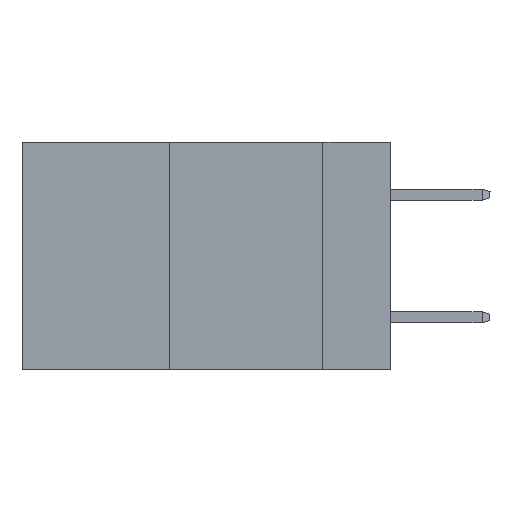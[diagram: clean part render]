
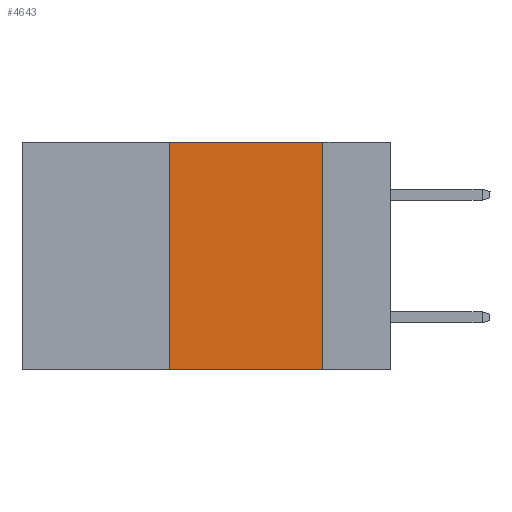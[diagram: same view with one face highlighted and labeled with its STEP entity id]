
A CAD part, left-side view. The second image highlights one B-rep face of the part: STEP entity #4643.
In plain terms, the highlighted planar face has unit normal (-1, 0, 0).
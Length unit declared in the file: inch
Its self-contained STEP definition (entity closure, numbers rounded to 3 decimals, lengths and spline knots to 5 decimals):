
#72 = DIRECTION ( 'NONE',  ( 0., -1., 0. ) ) ;
#659 = AXIS2_PLACEMENT_3D ( 'NONE', #6843, #3608, #16468 ) ;
#999 = CARTESIAN_POINT ( 'NONE',  ( 0., 0.36, -0.37 ) ) ;
#1176 = ORIENTED_EDGE ( 'NONE', *, *, #4001, .F. ) ;
#1846 = LINE ( 'NONE', #8462, #10432 ) ;
#2136 = VERTEX_POINT ( 'NONE', #12767 ) ;
#3608 = DIRECTION ( 'NONE',  ( 1., 0., 0. ) ) ;
#4001 = EDGE_CURVE ( 'NONE', #11012, #2136, #8260, .T. ) ;
#4234 = CARTESIAN_POINT ( 'NONE',  ( 0., 0.6, 0. ) ) ;
#4245 = EDGE_LOOP ( 'NONE', ( #16945, #1176, #9133, #13870 ) ) ;
#4643 = ADVANCED_FACE ( 'NONE', ( #8022 ), #15692, .F. ) ;
#5056 = VERTEX_POINT ( 'NONE', #999 ) ;
#5457 = VECTOR ( 'NONE', #6007, 39.37008 ) ;
#6007 = DIRECTION ( 'NONE',  ( 0., 0., -1. ) ) ;
#6843 = CARTESIAN_POINT ( 'NONE',  ( 0., 0.6, 0. ) ) ;
#6855 = DIRECTION ( 'NONE',  ( 0., 0., 1. ) ) ;
#7460 = DIRECTION ( 'NONE',  ( 0., -1., 0. ) ) ;
#8022 = FACE_OUTER_BOUND ( 'NONE', #4245, .T. ) ;
#8229 = EDGE_CURVE ( 'NONE', #2136, #10052, #17138, .T. ) ;
#8260 = LINE ( 'NONE', #4234, #12450 ) ;
#8462 = CARTESIAN_POINT ( 'NONE',  ( 0., 0.36, 0. ) ) ;
#9133 = ORIENTED_EDGE ( 'NONE', *, *, #12124, .F. ) ;
#10052 = VERTEX_POINT ( 'NONE', #12018 ) ;
#10432 = VECTOR ( 'NONE', #6855, 39.37008 ) ;
#11012 = VERTEX_POINT ( 'NONE', #11501 ) ;
#11501 = CARTESIAN_POINT ( 'NONE',  ( 0., 0.36, 0. ) ) ;
#12018 = CARTESIAN_POINT ( 'NONE',  ( 0., 0.11, -0.37 ) ) ;
#12124 = EDGE_CURVE ( 'NONE', #5056, #11012, #1846, .T. ) ;
#12450 = VECTOR ( 'NONE', #72, 39.37008 ) ;
#12767 = CARTESIAN_POINT ( 'NONE',  ( 0., 0.11, 0. ) ) ;
#13051 = CARTESIAN_POINT ( 'NONE',  ( 0., 0.11, 0. ) ) ;
#13870 = ORIENTED_EDGE ( 'NONE', *, *, #17488, .T. ) ;
#14575 = VECTOR ( 'NONE', #7460, 39.37008 ) ;
#15002 = LINE ( 'NONE', #16020, #14575 ) ;
#15692 = PLANE ( 'NONE',  #659 ) ;
#16020 = CARTESIAN_POINT ( 'NONE',  ( 0., 0.6, -0.37 ) ) ;
#16468 = DIRECTION ( 'NONE',  ( 0., 0., -1. ) ) ;
#16945 = ORIENTED_EDGE ( 'NONE', *, *, #8229, .F. ) ;
#17138 = LINE ( 'NONE', #13051, #5457 ) ;
#17488 = EDGE_CURVE ( 'NONE', #5056, #10052, #15002, .T. ) ;
